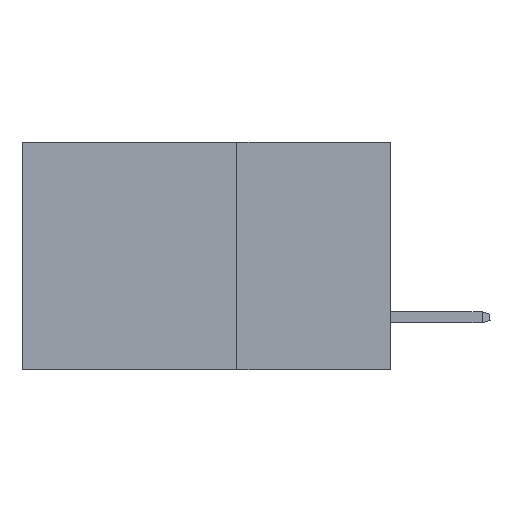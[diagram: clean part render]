
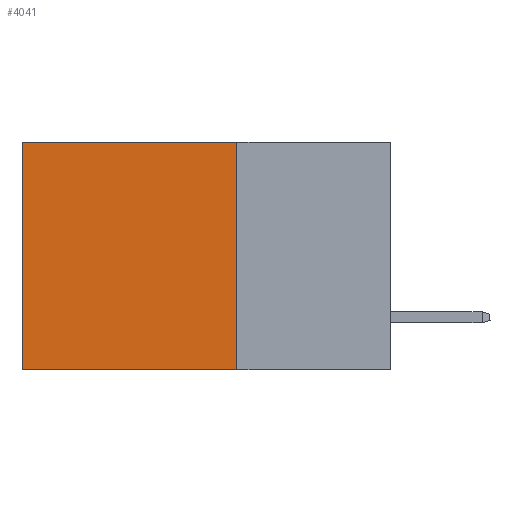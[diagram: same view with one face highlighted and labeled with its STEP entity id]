
A CAD part, left-side view. The second image highlights one B-rep face of the part: STEP entity #4041.
In plain terms, the highlighted planar face has unit normal (-1, 0, 0).
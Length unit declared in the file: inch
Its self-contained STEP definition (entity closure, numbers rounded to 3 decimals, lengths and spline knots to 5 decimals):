
#297 = VERTEX_POINT ( 'NONE', #3807 ) ;
#625 = DIRECTION ( 'NONE',  ( 0., 0., -1. ) ) ;
#825 = EDGE_CURVE ( 'NONE', #2447, #9951, #10683, .T. ) ;
#1918 = VECTOR ( 'NONE', #2841, 39.37008 ) ;
#2414 = LINE ( 'NONE', #5921, #1918 ) ;
#2447 = VERTEX_POINT ( 'NONE', #3594 ) ;
#2461 = CARTESIAN_POINT ( 'NONE',  ( 0.2875, 0.25, 0. ) ) ;
#2669 = CARTESIAN_POINT ( 'NONE',  ( 0.2875, 0.6, 0. ) ) ;
#2841 = DIRECTION ( 'NONE',  ( 0., 0., -1. ) ) ;
#3029 = FACE_OUTER_BOUND ( 'NONE', #12174, .T. ) ;
#3594 = CARTESIAN_POINT ( 'NONE',  ( 0.2875, 0.6, 0. ) ) ;
#3807 = CARTESIAN_POINT ( 'NONE',  ( 0.2875, 0.25, -0.37 ) ) ;
#4041 = ADVANCED_FACE ( 'NONE', ( #3029 ), #5813, .F. ) ;
#4651 = DIRECTION ( 'NONE',  ( 0., 0., -1. ) ) ;
#4756 = CARTESIAN_POINT ( 'NONE',  ( 0.2875, 0.25, 0. ) ) ;
#4928 = VECTOR ( 'NONE', #11989, 39.37008 ) ;
#5392 = VERTEX_POINT ( 'NONE', #10969 ) ;
#5759 = CARTESIAN_POINT ( 'NONE',  ( 0.2875, 0.25, -0.37 ) ) ;
#5813 = PLANE ( 'NONE',  #9502 ) ;
#5921 = CARTESIAN_POINT ( 'NONE',  ( 0.2875, 0.25, 0. ) ) ;
#6542 = ORIENTED_EDGE ( 'NONE', *, *, #9863, .F. ) ;
#6589 = ORIENTED_EDGE ( 'NONE', *, *, #7815, .F. ) ;
#6804 = DIRECTION ( 'NONE',  ( 0., 1., 0. ) ) ;
#6871 = DIRECTION ( 'NONE',  ( 1., 0., 0. ) ) ;
#7253 = VECTOR ( 'NONE', #6804, 39.37008 ) ;
#7727 = LINE ( 'NONE', #2461, #4928 ) ;
#7815 = EDGE_CURVE ( 'NONE', #297, #9951, #12052, .T. ) ;
#7877 = VECTOR ( 'NONE', #625, 39.37008 ) ;
#9502 = AXIS2_PLACEMENT_3D ( 'NONE', #4756, #6871, #4651 ) ;
#9518 = ORIENTED_EDGE ( 'NONE', *, *, #825, .T. ) ;
#9863 = EDGE_CURVE ( 'NONE', #5392, #297, #2414, .T. ) ;
#9951 = VERTEX_POINT ( 'NONE', #10108 ) ;
#10108 = CARTESIAN_POINT ( 'NONE',  ( 0.2875, 0.6, -0.37 ) ) ;
#10683 = LINE ( 'NONE', #2669, #7877 ) ;
#10969 = CARTESIAN_POINT ( 'NONE',  ( 0.2875, 0.25, 0. ) ) ;
#11307 = ORIENTED_EDGE ( 'NONE', *, *, #12981, .T. ) ;
#11989 = DIRECTION ( 'NONE',  ( 0., 1., 0. ) ) ;
#12052 = LINE ( 'NONE', #5759, #7253 ) ;
#12174 = EDGE_LOOP ( 'NONE', ( #9518, #6589, #6542, #11307 ) ) ;
#12981 = EDGE_CURVE ( 'NONE', #5392, #2447, #7727, .T. ) ;
